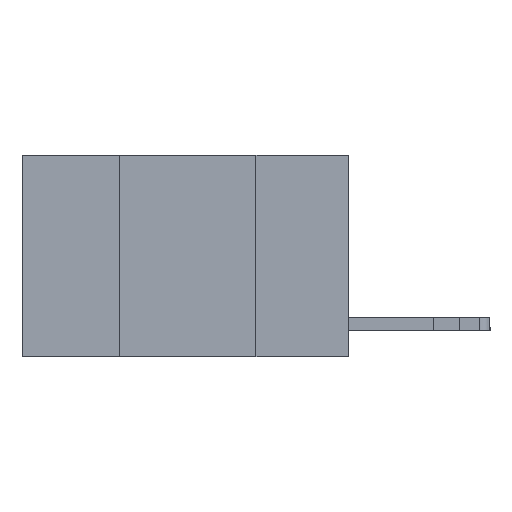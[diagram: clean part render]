
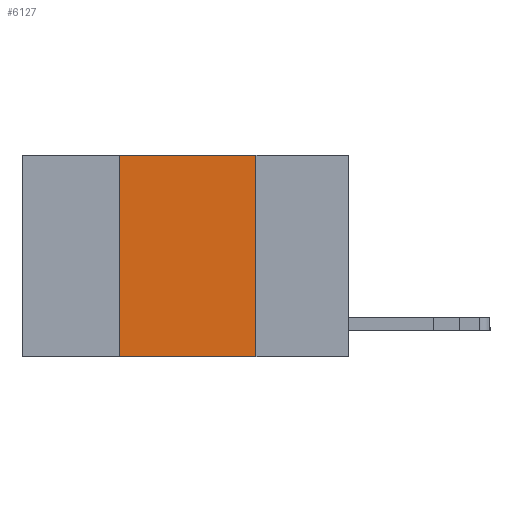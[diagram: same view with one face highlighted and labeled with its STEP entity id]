
A CAD part, left-side view. The second image highlights one B-rep face of the part: STEP entity #6127.
In plain terms, the highlighted planar face has unit normal (-1, 0, 0).
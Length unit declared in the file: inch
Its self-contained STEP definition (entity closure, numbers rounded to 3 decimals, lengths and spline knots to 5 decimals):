
#327 = EDGE_CURVE ( 'NONE', #4972, #11570, #979, .T. ) ;
#583 = EDGE_CURVE ( 'NONE', #8878, #9646, #3696, .T. ) ;
#979 = LINE ( 'NONE', #10401, #2414 ) ;
#1000 = DIRECTION ( 'NONE',  ( 0., -1., 0. ) ) ;
#1128 = VECTOR ( 'NONE', #5046, 39.37008 ) ;
#2414 = VECTOR ( 'NONE', #12665, 39.37008 ) ;
#2571 = EDGE_LOOP ( 'NONE', ( #8715, #4534, #4411, #12976 ) ) ;
#2812 = CARTESIAN_POINT ( 'NONE',  ( 0., 0.42, -0.37 ) ) ;
#3101 = EDGE_CURVE ( 'NONE', #4972, #9646, #8153, .T. ) ;
#3696 = LINE ( 'NONE', #7991, #7199 ) ;
#4277 = CARTESIAN_POINT ( 'NONE',  ( 0., 0.17, -0.37 ) ) ;
#4411 = ORIENTED_EDGE ( 'NONE', *, *, #327, .F. ) ;
#4534 = ORIENTED_EDGE ( 'NONE', *, *, #8286, .F. ) ;
#4972 = VERTEX_POINT ( 'NONE', #2812 ) ;
#5009 = CARTESIAN_POINT ( 'NONE',  ( 0., 0.6, 0. ) ) ;
#5046 = DIRECTION ( 'NONE',  ( 0., -1., 0. ) ) ;
#5552 = CARTESIAN_POINT ( 'NONE',  ( 0., 0.17, 0. ) ) ;
#5999 = DIRECTION ( 'NONE',  ( 0., 0., -1. ) ) ;
#6127 = ADVANCED_FACE ( 'NONE', ( #12100 ), #11069, .F. ) ;
#6162 = VECTOR ( 'NONE', #1000, 39.37008 ) ;
#6479 = AXIS2_PLACEMENT_3D ( 'NONE', #5009, #7271, #5999 ) ;
#7199 = VECTOR ( 'NONE', #7852, 39.37008 ) ;
#7271 = DIRECTION ( 'NONE',  ( 1., 0., 0. ) ) ;
#7852 = DIRECTION ( 'NONE',  ( 0., 0., -1. ) ) ;
#7991 = CARTESIAN_POINT ( 'NONE',  ( 0., 0.17, 0. ) ) ;
#8153 = LINE ( 'NONE', #9257, #6162 ) ;
#8286 = EDGE_CURVE ( 'NONE', #11570, #8878, #10339, .T. ) ;
#8715 = ORIENTED_EDGE ( 'NONE', *, *, #583, .F. ) ;
#8878 = VERTEX_POINT ( 'NONE', #5552 ) ;
#8918 = CARTESIAN_POINT ( 'NONE',  ( 0., 0.42, 0. ) ) ;
#9257 = CARTESIAN_POINT ( 'NONE',  ( 0., 0.6, -0.37 ) ) ;
#9646 = VERTEX_POINT ( 'NONE', #4277 ) ;
#10339 = LINE ( 'NONE', #11366, #1128 ) ;
#10401 = CARTESIAN_POINT ( 'NONE',  ( 0., 0.42, 0. ) ) ;
#11069 = PLANE ( 'NONE',  #6479 ) ;
#11366 = CARTESIAN_POINT ( 'NONE',  ( 0., 0.6, 0. ) ) ;
#11570 = VERTEX_POINT ( 'NONE', #8918 ) ;
#12100 = FACE_OUTER_BOUND ( 'NONE', #2571, .T. ) ;
#12665 = DIRECTION ( 'NONE',  ( 0., 0., 1. ) ) ;
#12976 = ORIENTED_EDGE ( 'NONE', *, *, #3101, .T. ) ;
